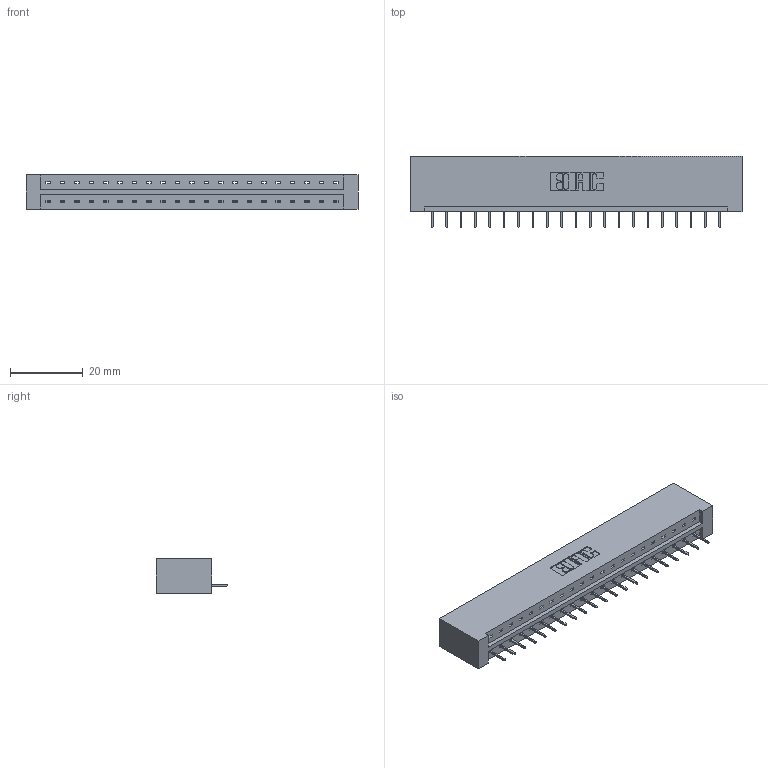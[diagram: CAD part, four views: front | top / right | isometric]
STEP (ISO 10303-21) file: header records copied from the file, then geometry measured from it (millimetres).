
FILE_DESCRIPTION (( 'STEP AP203' ), '1' );
FILE_NAME ('333-021-524-101.STEP', '2018-08-02T01:02:49', ( '' ), ( '' ), 'SwSTEP 2.0', 'SolidWorks 2016', '' );
FILE_SCHEMA (( 'CONFIG_CONTROL_DESIGN' ));
Length unit declared in the file: inch
Products named in the file (3): 333-021-524-101; 333 Part_Lugless; 345-292-001_345-293-124
Assembly tree (22 placements, depth 2):
  333-021-524-101
    333 Part_Lugless
    345-292-001_345-293-124  x21
Bounding box: 91.47 x 19.69 x 9.4 mm (x, y, z)
Volume: 9553.2 mm3; surface area: 9870.4 mm2
Topology: 22 solids, 22 shells, 1408 faces, 4067 edges, 2626 vertices
Faces by surface type: plane 1074, cylinder 334
Entity records: 15351 total; most frequent: CARTESIAN_POINT 2657, ORIENTED_EDGE 2614, DIRECTION 2277, EDGE_CURVE 1307, LINE 1191, VECTOR 1191, VERTEX_POINT 866, AXIS2_PLACEMENT_3D 543
